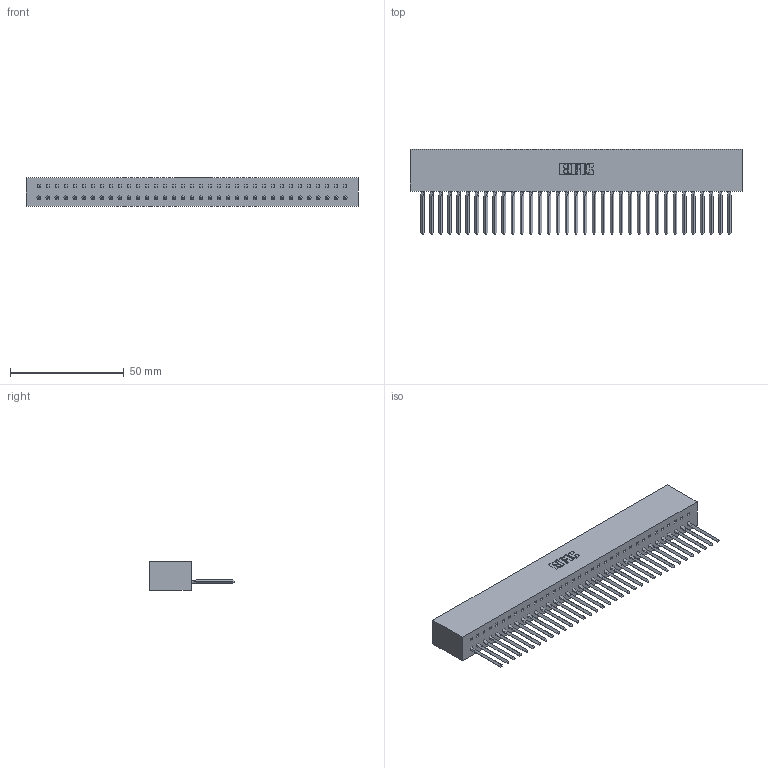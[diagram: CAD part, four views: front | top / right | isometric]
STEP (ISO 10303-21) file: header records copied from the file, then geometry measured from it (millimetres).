
FILE_DESCRIPTION (( 'STEP AP203' ), '1' );
FILE_NAME ('317-035-541-601.STEP', '2020-02-27T22:20:28', ( '' ), ( '' ), 'SwSTEP 2.0', 'SolidWorks 2016', '' );
FILE_SCHEMA (( 'CONFIG_CONTROL_DESIGN' ));
Length unit declared in the file: inch
Products named in the file (3): 317-290-002_541; 317-035-541-601; 317 Part_Lugless
Assembly tree (36 placements, depth 2):
  317-035-541-601
    317 Part_Lugless
    317-290-002_541  x35
Bounding box: 145.9 x 37.34 x 12.7 mm (x, y, z)
Volume: 25150.3 mm3; surface area: 35499.3 mm2
Topology: 36 solids, 36 shells, 5410 faces, 15429 edges, 10028 vertices
Faces by surface type: plane 4390, cylinder 880, bspline 140
Entity records: 51588 total; most frequent: CARTESIAN_POINT 9810, ORIENTED_EDGE 9098, DIRECTION 7459, EDGE_CURVE 4549, VECTOR 4193, LINE 4193, VERTEX_POINT 3024, AXIS2_PLACEMENT_3D 1633
